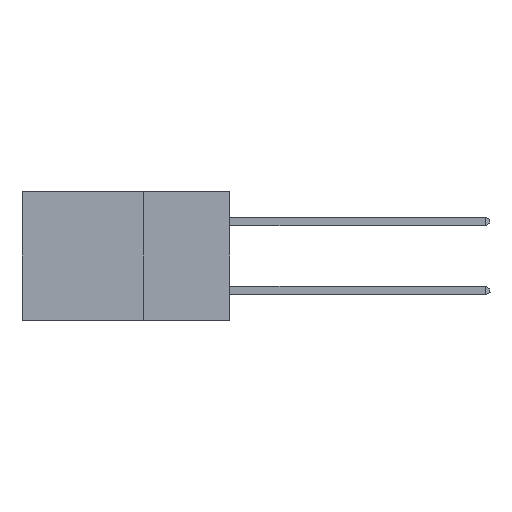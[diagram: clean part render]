
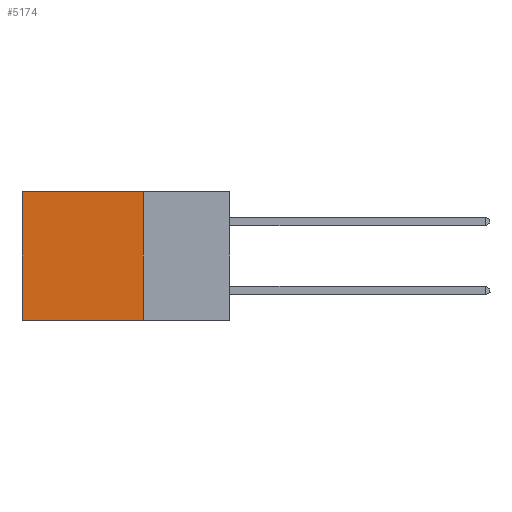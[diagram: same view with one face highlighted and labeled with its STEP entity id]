
A CAD part, left-side view. The second image highlights one B-rep face of the part: STEP entity #5174.
In plain terms, the highlighted planar face has unit normal (-1, 0, 0).
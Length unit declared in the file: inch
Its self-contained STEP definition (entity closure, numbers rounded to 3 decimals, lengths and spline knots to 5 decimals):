
#132 = FACE_OUTER_BOUND ( 'NONE', #11278, .T. ) ;
#713 = VERTEX_POINT ( 'NONE', #18240 ) ;
#1779 = CARTESIAN_POINT ( 'NONE',  ( 0.298, 0.25, 0. ) ) ;
#2713 = ORIENTED_EDGE ( 'NONE', *, *, #11476, .T. ) ;
#3157 = AXIS2_PLACEMENT_3D ( 'NONE', #16481, #8225, #19771 ) ;
#3716 = CARTESIAN_POINT ( 'NONE',  ( 0.298, 0.25, 0. ) ) ;
#4863 = EDGE_CURVE ( 'NONE', #10607, #15425, #15117, .T. ) ;
#5174 = ADVANCED_FACE ( 'NONE', ( #132 ), #6581, .F. ) ;
#5346 = CARTESIAN_POINT ( 'NONE',  ( 0.298, 0.6, -0.37 ) ) ;
#5371 = DIRECTION ( 'NONE',  ( 0., 1., 0. ) ) ;
#5764 = CARTESIAN_POINT ( 'NONE',  ( 0.298, 0.25, 0. ) ) ;
#6581 = PLANE ( 'NONE',  #3157 ) ;
#7546 = VECTOR ( 'NONE', #11710, 39.37008 ) ;
#8225 = DIRECTION ( 'NONE',  ( 1., 0., 0. ) ) ;
#8412 = LINE ( 'NONE', #3716, #12834 ) ;
#8525 = VECTOR ( 'NONE', #11672, 39.37008 ) ;
#10015 = CARTESIAN_POINT ( 'NONE',  ( 0.298, 0.6, 0. ) ) ;
#10607 = VERTEX_POINT ( 'NONE', #15988 ) ;
#10692 = DIRECTION ( 'NONE',  ( 0., 1., 0. ) ) ;
#10716 = VECTOR ( 'NONE', #10692, 39.37008 ) ;
#11278 = EDGE_LOOP ( 'NONE', ( #2713, #20962, #12807, #15956 ) ) ;
#11476 = EDGE_CURVE ( 'NONE', #713, #15425, #11989, .T. ) ;
#11672 = DIRECTION ( 'NONE',  ( 0., 0., -1. ) ) ;
#11710 = DIRECTION ( 'NONE',  ( 0., 0., -1. ) ) ;
#11989 = LINE ( 'NONE', #10015, #7546 ) ;
#12759 = EDGE_CURVE ( 'NONE', #17249, #10607, #21151, .T. ) ;
#12807 = ORIENTED_EDGE ( 'NONE', *, *, #12759, .F. ) ;
#12834 = VECTOR ( 'NONE', #5371, 39.37008 ) ;
#13966 = CARTESIAN_POINT ( 'NONE',  ( 0.298, 0.25, -0.37 ) ) ;
#15117 = LINE ( 'NONE', #13966, #10716 ) ;
#15425 = VERTEX_POINT ( 'NONE', #5346 ) ;
#15956 = ORIENTED_EDGE ( 'NONE', *, *, #19725, .T. ) ;
#15988 = CARTESIAN_POINT ( 'NONE',  ( 0.298, 0.25, -0.37 ) ) ;
#16481 = CARTESIAN_POINT ( 'NONE',  ( 0.298, 0.25, 0. ) ) ;
#17249 = VERTEX_POINT ( 'NONE', #5764 ) ;
#18240 = CARTESIAN_POINT ( 'NONE',  ( 0.298, 0.6, 0. ) ) ;
#19725 = EDGE_CURVE ( 'NONE', #17249, #713, #8412, .T. ) ;
#19771 = DIRECTION ( 'NONE',  ( 0., 0., -1. ) ) ;
#20962 = ORIENTED_EDGE ( 'NONE', *, *, #4863, .F. ) ;
#21151 = LINE ( 'NONE', #1779, #8525 ) ;
